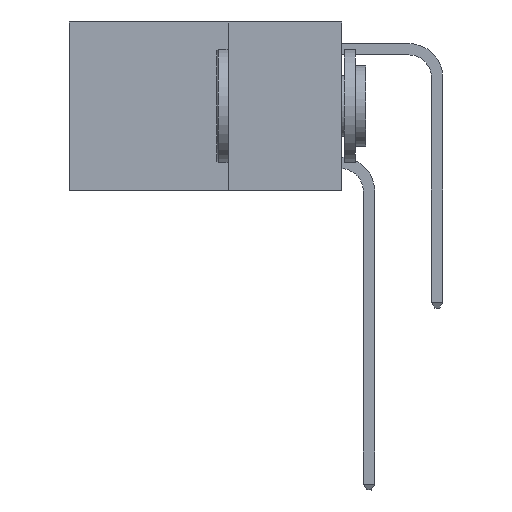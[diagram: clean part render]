
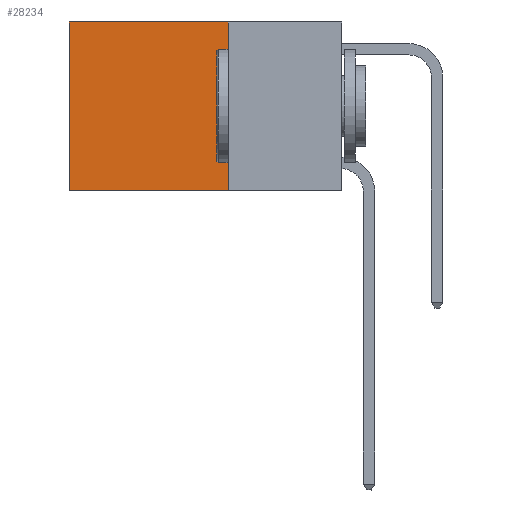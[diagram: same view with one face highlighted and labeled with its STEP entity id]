
A CAD part, left-side view. The second image highlights one B-rep face of the part: STEP entity #28234.
In plain terms, the highlighted planar face has unit normal (-1, 0, 0).
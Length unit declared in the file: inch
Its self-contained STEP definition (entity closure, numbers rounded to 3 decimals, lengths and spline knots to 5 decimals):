
#277 = CARTESIAN_POINT ( 'NONE',  ( 0.2625, 0.6, 0. ) ) ;
#323 = CARTESIAN_POINT ( 'NONE',  ( 0.2625, 0.25, -0.37 ) ) ;
#1244 = ORIENTED_EDGE ( 'NONE', *, *, #13867, .T. ) ;
#1428 = DIRECTION ( 'NONE',  ( 0., 0., -1. ) ) ;
#1627 = VECTOR ( 'NONE', #11135, 39.37008 ) ;
#3742 = VERTEX_POINT ( 'NONE', #4456 ) ;
#4239 = CARTESIAN_POINT ( 'NONE',  ( 0.2625, 0.25, 0. ) ) ;
#4456 = CARTESIAN_POINT ( 'NONE',  ( 0.2625, 0.25, 0. ) ) ;
#4701 = EDGE_LOOP ( 'NONE', ( #15796, #9830, #9911, #1244 ) ) ;
#5395 = LINE ( 'NONE', #12516, #23394 ) ;
#5443 = DIRECTION ( 'NONE',  ( 0., 1., 0. ) ) ;
#6602 = DIRECTION ( 'NONE',  ( 1., 0., 0. ) ) ;
#6941 = VERTEX_POINT ( 'NONE', #323 ) ;
#7175 = LINE ( 'NONE', #22834, #1627 ) ;
#7819 = FACE_OUTER_BOUND ( 'NONE', #4701, .T. ) ;
#8715 = DIRECTION ( 'NONE',  ( 0., 0., -1. ) ) ;
#9830 = ORIENTED_EDGE ( 'NONE', *, *, #15671, .F. ) ;
#9911 = ORIENTED_EDGE ( 'NONE', *, *, #25729, .F. ) ;
#11135 = DIRECTION ( 'NONE',  ( 0., 1., 0. ) ) ;
#12516 = CARTESIAN_POINT ( 'NONE',  ( 0.2625, 0.25, 0. ) ) ;
#13867 = EDGE_CURVE ( 'NONE', #3742, #19351, #5395, .T. ) ;
#14433 = LINE ( 'NONE', #22778, #21417 ) ;
#15671 = EDGE_CURVE ( 'NONE', #6941, #28887, #7175, .T. ) ;
#15796 = ORIENTED_EDGE ( 'NONE', *, *, #30345, .T. ) ;
#17800 = CARTESIAN_POINT ( 'NONE',  ( 0.2625, 0.6, 0. ) ) ;
#18040 = LINE ( 'NONE', #17800, #29705 ) ;
#18313 = PLANE ( 'NONE',  #26744 ) ;
#19351 = VERTEX_POINT ( 'NONE', #277 ) ;
#20543 = CARTESIAN_POINT ( 'NONE',  ( 0.2625, 0.6, -0.37 ) ) ;
#21417 = VECTOR ( 'NONE', #8715, 39.37008 ) ;
#22778 = CARTESIAN_POINT ( 'NONE',  ( 0.2625, 0.25, 0. ) ) ;
#22834 = CARTESIAN_POINT ( 'NONE',  ( 0.2625, 0.25, -0.37 ) ) ;
#23033 = DIRECTION ( 'NONE',  ( 0., 0., -1. ) ) ;
#23394 = VECTOR ( 'NONE', #5443, 39.37008 ) ;
#25729 = EDGE_CURVE ( 'NONE', #3742, #6941, #14433, .T. ) ;
#26744 = AXIS2_PLACEMENT_3D ( 'NONE', #4239, #6602, #23033 ) ;
#28234 = ADVANCED_FACE ( 'NONE', ( #7819 ), #18313, .F. ) ;
#28887 = VERTEX_POINT ( 'NONE', #20543 ) ;
#29705 = VECTOR ( 'NONE', #1428, 39.37008 ) ;
#30345 = EDGE_CURVE ( 'NONE', #19351, #28887, #18040, .T. ) ;
